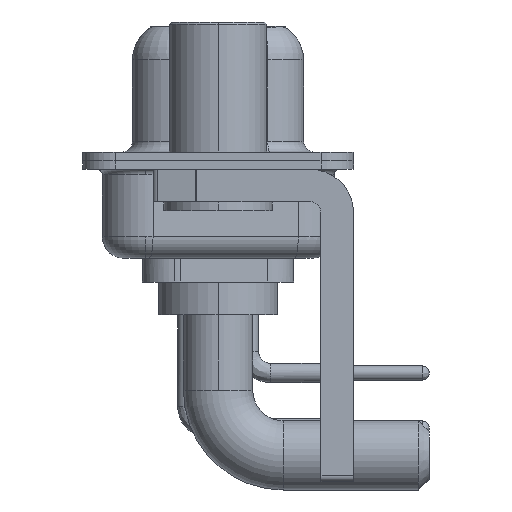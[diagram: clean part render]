
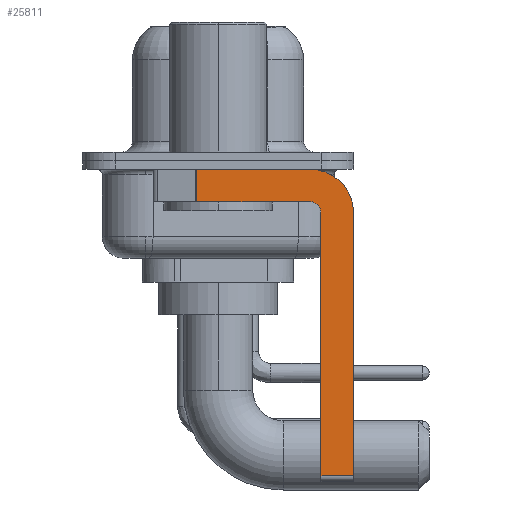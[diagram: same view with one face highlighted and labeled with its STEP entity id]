
A CAD part, left-side view. The second image highlights one B-rep face of the part: STEP entity #25811.
In plain terms, the highlighted planar face has unit normal (-1, 0, 0).
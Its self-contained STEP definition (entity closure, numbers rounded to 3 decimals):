
#216 = DIRECTION ( 'NONE',  ( -1., 0., 0. ) ) ;
#629 = EDGE_CURVE ( 'NONE', #9929, #10741, #3779, .T. ) ;
#837 = CARTESIAN_POINT ( 'NONE',  ( -2.9, -4.75, -2.4 ) ) ;
#872 = CARTESIAN_POINT ( 'NONE',  ( -2.9, -4.75, -14.55 ) ) ;
#965 = ORIENTED_EDGE ( 'NONE', *, *, #18447, .F. ) ;
#1191 = LINE ( 'NONE', #5212, #12042 ) ;
#1501 = CARTESIAN_POINT ( 'NONE',  ( -2.9, -4.25, -1.9 ) ) ;
#2029 = DIRECTION ( 'NONE',  ( 0., 0., -1. ) ) ;
#2096 = VERTEX_POINT ( 'NONE', #837 ) ;
#2303 = DIRECTION ( 'NONE',  ( 0., 0., 1. ) ) ;
#2721 = VECTOR ( 'NONE', #9668, 1000. ) ;
#2941 = ORIENTED_EDGE ( 'NONE', *, *, #10264, .T. ) ;
#3009 = VERTEX_POINT ( 'NONE', #872 ) ;
#3779 = LINE ( 'NONE', #12493, #22486 ) ;
#3914 = EDGE_LOOP ( 'NONE', ( #7127, #23762, #14417, #15026, #23169, #2941, #965, #22485 ) ) ;
#3920 = DIRECTION ( 'NONE',  ( 0., 1., 0. ) ) ;
#4403 = VECTOR ( 'NONE', #6770, 1000. ) ;
#5212 = CARTESIAN_POINT ( 'NONE',  ( -2.9, -4.75, -14.8 ) ) ;
#6602 = VERTEX_POINT ( 'NONE', #13225 ) ;
#6770 = DIRECTION ( 'NONE',  ( 0., 0., -1. ) ) ;
#7127 = ORIENTED_EDGE ( 'NONE', *, *, #21893, .F. ) ;
#7293 = CARTESIAN_POINT ( 'NONE',  ( -2.9, 0.978, -1.9 ) ) ;
#7867 = LINE ( 'NONE', #26946, #2721 ) ;
#8368 = CARTESIAN_POINT ( 'NONE',  ( -2.9, 0.978, -1.9 ) ) ;
#9668 = DIRECTION ( 'NONE',  ( 0., -1., 0. ) ) ;
#9706 = CARTESIAN_POINT ( 'NONE',  ( -2.9, -4.25, -2.4 ) ) ;
#9929 = VERTEX_POINT ( 'NONE', #1501 ) ;
#10264 = EDGE_CURVE ( 'NONE', #3009, #20530, #11578, .T. ) ;
#10741 = VERTEX_POINT ( 'NONE', #7293 ) ;
#11052 = LINE ( 'NONE', #15216, #4403 ) ;
#11578 = LINE ( 'NONE', #13933, #18898 ) ;
#12042 = VECTOR ( 'NONE', #13938, 1000. ) ;
#12493 = CARTESIAN_POINT ( 'NONE',  ( -2.9, -4.25, -1.9 ) ) ;
#13097 = EDGE_CURVE ( 'NONE', #6602, #13178, #25231, .T. ) ;
#13178 = VERTEX_POINT ( 'NONE', #18905 ) ;
#13225 = CARTESIAN_POINT ( 'NONE',  ( -2.9, -4.25, -0.4 ) ) ;
#13244 = VERTEX_POINT ( 'NONE', #25814 ) ;
#13281 = EDGE_CURVE ( 'NONE', #2096, #9929, #19475, .T. ) ;
#13483 = FACE_OUTER_BOUND ( 'NONE', #3914, .T. ) ;
#13933 = CARTESIAN_POINT ( 'NONE',  ( -2.9, -4.25, -14.55 ) ) ;
#13938 = DIRECTION ( 'NONE',  ( 0., 0., 1. ) ) ;
#14225 = CARTESIAN_POINT ( 'NONE',  ( -2.9, -4.25, -2.4 ) ) ;
#14417 = ORIENTED_EDGE ( 'NONE', *, *, #629, .F. ) ;
#14498 = DIRECTION ( 'NONE',  ( 1., 0., 0. ) ) ;
#14608 = VECTOR ( 'NONE', #25795, 1000. ) ;
#15026 = ORIENTED_EDGE ( 'NONE', *, *, #13281, .F. ) ;
#15216 = CARTESIAN_POINT ( 'NONE',  ( -2.9, -6.25, -2.4 ) ) ;
#17619 = PLANE ( 'NONE',  #18064 ) ;
#18064 = AXIS2_PLACEMENT_3D ( 'NONE', #9706, #26572, #23987 ) ;
#18447 = EDGE_CURVE ( 'NONE', #13178, #20530, #11052, .T. ) ;
#18745 = CARTESIAN_POINT ( 'NONE',  ( -2.9, -6.25, -14.55 ) ) ;
#18898 = VECTOR ( 'NONE', #24288, 1000. ) ;
#18905 = CARTESIAN_POINT ( 'NONE',  ( -2.9, -6.25, -2.4 ) ) ;
#19475 = CIRCLE ( 'NONE', #25250, 0.5 ) ;
#20530 = VERTEX_POINT ( 'NONE', #18745 ) ;
#20577 = EDGE_CURVE ( 'NONE', #13244, #10741, #23017, .T. ) ;
#21893 = EDGE_CURVE ( 'NONE', #13244, #6602, #7867, .T. ) ;
#22363 = EDGE_CURVE ( 'NONE', #3009, #2096, #1191, .T. ) ;
#22485 = ORIENTED_EDGE ( 'NONE', *, *, #13097, .F. ) ;
#22486 = VECTOR ( 'NONE', #3920, 1000. ) ;
#23017 = LINE ( 'NONE', #8368, #14608 ) ;
#23169 = ORIENTED_EDGE ( 'NONE', *, *, #22363, .F. ) ;
#23715 = CARTESIAN_POINT ( 'NONE',  ( -2.9, -4.25, -2.4 ) ) ;
#23762 = ORIENTED_EDGE ( 'NONE', *, *, #20577, .T. ) ;
#23987 = DIRECTION ( 'NONE',  ( 0., 0., -1. ) ) ;
#24288 = DIRECTION ( 'NONE',  ( 0., -1., 0. ) ) ;
#25231 = CIRCLE ( 'NONE', #26085, 2. ) ;
#25250 = AXIS2_PLACEMENT_3D ( 'NONE', #23715, #216, #2303 ) ;
#25795 = DIRECTION ( 'NONE',  ( 0., 0., -1. ) ) ;
#25811 = ADVANCED_FACE ( 'NONE', ( #13483 ), #17619, .F. ) ;
#25814 = CARTESIAN_POINT ( 'NONE',  ( -2.9, 0.978, -0.4 ) ) ;
#26085 = AXIS2_PLACEMENT_3D ( 'NONE', #14225, #14498, #2029 ) ;
#26572 = DIRECTION ( 'NONE',  ( 1., 0., 0. ) ) ;
#26946 = CARTESIAN_POINT ( 'NONE',  ( -2.9, 3., -0.4 ) ) ;
